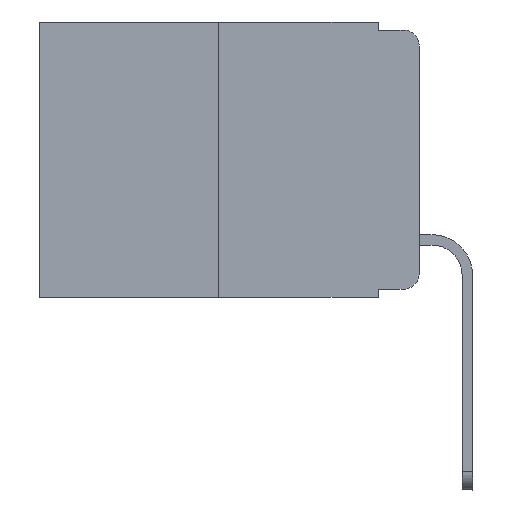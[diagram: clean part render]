
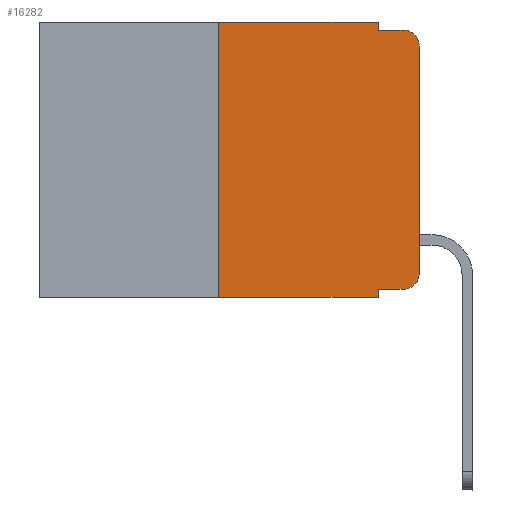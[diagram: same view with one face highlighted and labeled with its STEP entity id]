
A CAD part, left-side view. The second image highlights one B-rep face of the part: STEP entity #16282.
In plain terms, the highlighted planar face has unit normal (-1, 0, 0).
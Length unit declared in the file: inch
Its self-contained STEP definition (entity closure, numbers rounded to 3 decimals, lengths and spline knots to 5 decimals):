
#64 = VERTEX_POINT ( 'NONE', #15902 ) ;
#178 = ORIENTED_EDGE ( 'NONE', *, *, #14572, .T. ) ;
#653 = VERTEX_POINT ( 'NONE', #8318 ) ;
#760 = VECTOR ( 'NONE', #10054, 39.37008 ) ;
#1112 = VERTEX_POINT ( 'NONE', #17513 ) ;
#1671 = LINE ( 'NONE', #4441, #17489 ) ;
#1792 = VERTEX_POINT ( 'NONE', #10823 ) ;
#2026 = EDGE_CURVE ( 'NONE', #9091, #1112, #17536, .T. ) ;
#2084 = CARTESIAN_POINT ( 'NONE',  ( 0., 0.473, 0. ) ) ;
#2425 = ORIENTED_EDGE ( 'NONE', *, *, #3277, .T. ) ;
#2532 = PLANE ( 'NONE',  #6881 ) ;
#2567 = VECTOR ( 'NONE', #16819, 39.37008 ) ;
#3222 = EDGE_CURVE ( 'NONE', #1792, #653, #4099, .T. ) ;
#3277 = EDGE_CURVE ( 'NONE', #10505, #5627, #14045, .T. ) ;
#3315 = ORIENTED_EDGE ( 'NONE', *, *, #2026, .T. ) ;
#3861 = EDGE_CURVE ( 'NONE', #9091, #5627, #6097, .T. ) ;
#4099 = CIRCLE ( 'NONE', #12071, 0.02 ) ;
#4240 = VECTOR ( 'NONE', #14488, 39.37008 ) ;
#4425 = VECTOR ( 'NONE', #15603, 39.37008 ) ;
#4441 = CARTESIAN_POINT ( 'NONE',  ( 0., 0.25, 0. ) ) ;
#4762 = CIRCLE ( 'NONE', #6294, 0.02 ) ;
#4894 = ORIENTED_EDGE ( 'NONE', *, *, #9369, .T. ) ;
#4980 = EDGE_CURVE ( 'NONE', #10505, #11966, #1671, .T. ) ;
#5328 = CARTESIAN_POINT ( 'NONE',  ( 0., 0.051, -0.01 ) ) ;
#5463 = VECTOR ( 'NONE', #5482, 39.37008 ) ;
#5482 = DIRECTION ( 'NONE',  ( 0., 0., -1. ) ) ;
#5627 = VERTEX_POINT ( 'NONE', #18325 ) ;
#6097 = LINE ( 'NONE', #11958, #760 ) ;
#6101 = VECTOR ( 'NONE', #8019, 39.37008 ) ;
#6294 = AXIS2_PLACEMENT_3D ( 'NONE', #8219, #15712, #11297 ) ;
#6570 = FACE_OUTER_BOUND ( 'NONE', #13048, .T. ) ;
#6881 = AXIS2_PLACEMENT_3D ( 'NONE', #17038, #15699, #14266 ) ;
#6888 = ORIENTED_EDGE ( 'NONE', *, *, #13730, .F. ) ;
#7166 = EDGE_CURVE ( 'NONE', #9303, #653, #17840, .T. ) ;
#7522 = DIRECTION ( 'NONE',  ( 0., 0., 1. ) ) ;
#8019 = DIRECTION ( 'NONE',  ( 0., -1., 0. ) ) ;
#8219 = CARTESIAN_POINT ( 'NONE',  ( 0., 0.02, -0.313 ) ) ;
#8318 = CARTESIAN_POINT ( 'NONE',  ( 0., 0.02, -0.01 ) ) ;
#8554 = CARTESIAN_POINT ( 'NONE',  ( 0., 0., -0.313 ) ) ;
#8980 = ORIENTED_EDGE ( 'NONE', *, *, #7166, .F. ) ;
#9091 = VERTEX_POINT ( 'NONE', #17382 ) ;
#9303 = VERTEX_POINT ( 'NONE', #5328 ) ;
#9369 = EDGE_CURVE ( 'NONE', #1112, #13706, #4762, .T. ) ;
#9523 = DIRECTION ( 'NONE',  ( 0., 0., -1. ) ) ;
#9708 = DIRECTION ( 'NONE',  ( -1., 0., 0. ) ) ;
#10004 = LINE ( 'NONE', #11144, #5463 ) ;
#10054 = DIRECTION ( 'NONE',  ( 0., 0., -1. ) ) ;
#10505 = VERTEX_POINT ( 'NONE', #10558 ) ;
#10558 = CARTESIAN_POINT ( 'NONE',  ( 0., 0.25, -0.343 ) ) ;
#10737 = DIRECTION ( 'NONE',  ( 0., -1., 0. ) ) ;
#10823 = CARTESIAN_POINT ( 'NONE',  ( 0., 0., -0.03 ) ) ;
#10947 = CARTESIAN_POINT ( 'NONE',  ( 0., 0.02, -0.03 ) ) ;
#11144 = CARTESIAN_POINT ( 'NONE',  ( 0., 0.051, 0. ) ) ;
#11297 = DIRECTION ( 'NONE',  ( 0., 0., -1. ) ) ;
#11958 = CARTESIAN_POINT ( 'NONE',  ( 0., 0.051, 0. ) ) ;
#11966 = VERTEX_POINT ( 'NONE', #18499 ) ;
#12071 = AXIS2_PLACEMENT_3D ( 'NONE', #10947, #9708, #9523 ) ;
#12680 = EDGE_CURVE ( 'NONE', #11966, #64, #13905, .T. ) ;
#12830 = LINE ( 'NONE', #17130, #4425 ) ;
#13048 = EDGE_LOOP ( 'NONE', ( #178, #15475, #8980, #6888, #13888, #14830, #2425, #17200, #3315, #4894 ) ) ;
#13153 = CARTESIAN_POINT ( 'NONE',  ( 0., 0.051, -0.333 ) ) ;
#13706 = VERTEX_POINT ( 'NONE', #8554 ) ;
#13730 = EDGE_CURVE ( 'NONE', #64, #9303, #10004, .T. ) ;
#13888 = ORIENTED_EDGE ( 'NONE', *, *, #12680, .F. ) ;
#13905 = LINE ( 'NONE', #2084, #6101 ) ;
#13941 = CARTESIAN_POINT ( 'NONE',  ( 0., 0.473, -0.343 ) ) ;
#14045 = LINE ( 'NONE', #13941, #2567 ) ;
#14266 = DIRECTION ( 'NONE',  ( 0., 0., -1. ) ) ;
#14488 = DIRECTION ( 'NONE',  ( 0., -1., 0. ) ) ;
#14572 = EDGE_CURVE ( 'NONE', #13706, #1792, #12830, .T. ) ;
#14830 = ORIENTED_EDGE ( 'NONE', *, *, #4980, .F. ) ;
#15475 = ORIENTED_EDGE ( 'NONE', *, *, #3222, .T. ) ;
#15603 = DIRECTION ( 'NONE',  ( 0., 0., 1. ) ) ;
#15699 = DIRECTION ( 'NONE',  ( 1., 0., 0. ) ) ;
#15712 = DIRECTION ( 'NONE',  ( -1., 0., 0. ) ) ;
#15902 = CARTESIAN_POINT ( 'NONE',  ( 0., 0.051, 0. ) ) ;
#16282 = ADVANCED_FACE ( 'NONE', ( #6570 ), #2532, .F. ) ;
#16318 = CARTESIAN_POINT ( 'NONE',  ( 0., 0.051, -0.01 ) ) ;
#16819 = DIRECTION ( 'NONE',  ( 0., -1., 0. ) ) ;
#17038 = CARTESIAN_POINT ( 'NONE',  ( 0., 0.473, 0. ) ) ;
#17130 = CARTESIAN_POINT ( 'NONE',  ( 0., 0., 0. ) ) ;
#17200 = ORIENTED_EDGE ( 'NONE', *, *, #3861, .F. ) ;
#17382 = CARTESIAN_POINT ( 'NONE',  ( 0., 0.051, -0.333 ) ) ;
#17489 = VECTOR ( 'NONE', #7522, 39.37008 ) ;
#17513 = CARTESIAN_POINT ( 'NONE',  ( 0., 0.02, -0.333 ) ) ;
#17536 = LINE ( 'NONE', #13153, #4240 ) ;
#17771 = VECTOR ( 'NONE', #10737, 39.37008 ) ;
#17840 = LINE ( 'NONE', #16318, #17771 ) ;
#18325 = CARTESIAN_POINT ( 'NONE',  ( 0., 0.051, -0.343 ) ) ;
#18499 = CARTESIAN_POINT ( 'NONE',  ( 0., 0.25, 0. ) ) ;
